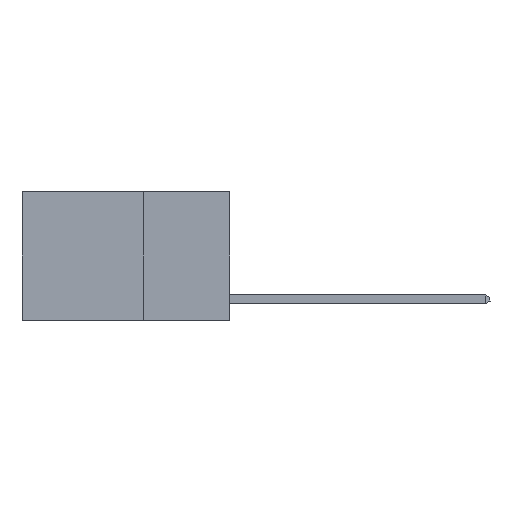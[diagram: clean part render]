
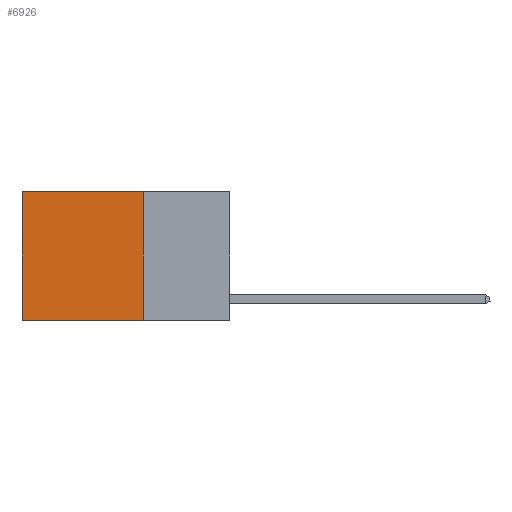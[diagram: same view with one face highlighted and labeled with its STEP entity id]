
A CAD part, left-side view. The second image highlights one B-rep face of the part: STEP entity #6926.
In plain terms, the highlighted planar face has unit normal (-1, 0, 0).
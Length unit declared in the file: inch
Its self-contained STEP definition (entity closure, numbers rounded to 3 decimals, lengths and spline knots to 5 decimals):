
#720 = LINE ( 'NONE', #11697, #869 ) ;
#869 = VECTOR ( 'NONE', #1500, 39.37008 ) ;
#1333 = LINE ( 'NONE', #8462, #12494 ) ;
#1369 = PLANE ( 'NONE',  #10011 ) ;
#1450 = DIRECTION ( 'NONE',  ( 0., 0., -1. ) ) ;
#1488 = LINE ( 'NONE', #3428, #2907 ) ;
#1500 = DIRECTION ( 'NONE',  ( 0., 0., -1. ) ) ;
#1533 = CARTESIAN_POINT ( 'NONE',  ( 0.2625, 0.25, 0. ) ) ;
#1823 = EDGE_CURVE ( 'NONE', #12910, #5842, #720, .T. ) ;
#2907 = VECTOR ( 'NONE', #11552, 39.37008 ) ;
#3292 = EDGE_CURVE ( 'NONE', #6196, #12910, #1488, .T. ) ;
#3428 = CARTESIAN_POINT ( 'NONE',  ( 0.2625, 0.25, 0. ) ) ;
#3432 = CARTESIAN_POINT ( 'NONE',  ( 0.2625, 0.25, 0. ) ) ;
#3776 = CARTESIAN_POINT ( 'NONE',  ( 0.2625, 0.6, 0. ) ) ;
#4314 = VECTOR ( 'NONE', #1450, 39.37008 ) ;
#4449 = CARTESIAN_POINT ( 'NONE',  ( 0.2625, 0.25, 0. ) ) ;
#5058 = CARTESIAN_POINT ( 'NONE',  ( 0.2625, 0.25, -0.37 ) ) ;
#5737 = ORIENTED_EDGE ( 'NONE', *, *, #1823, .T. ) ;
#5842 = VERTEX_POINT ( 'NONE', #6462 ) ;
#6196 = VERTEX_POINT ( 'NONE', #1533 ) ;
#6462 = CARTESIAN_POINT ( 'NONE',  ( 0.2625, 0.6, -0.37 ) ) ;
#6736 = EDGE_LOOP ( 'NONE', ( #5737, #9931, #10718, #8249 ) ) ;
#6926 = ADVANCED_FACE ( 'NONE', ( #11349 ), #1369, .F. ) ;
#8249 = ORIENTED_EDGE ( 'NONE', *, *, #3292, .T. ) ;
#8462 = CARTESIAN_POINT ( 'NONE',  ( 0.2625, 0.25, -0.37 ) ) ;
#9570 = EDGE_CURVE ( 'NONE', #6196, #11566, #12366, .T. ) ;
#9606 = EDGE_CURVE ( 'NONE', #11566, #5842, #1333, .T. ) ;
#9931 = ORIENTED_EDGE ( 'NONE', *, *, #9606, .F. ) ;
#10011 = AXIS2_PLACEMENT_3D ( 'NONE', #3432, #12468, #12406 ) ;
#10718 = ORIENTED_EDGE ( 'NONE', *, *, #9570, .F. ) ;
#11185 = DIRECTION ( 'NONE',  ( 0., 1., 0. ) ) ;
#11349 = FACE_OUTER_BOUND ( 'NONE', #6736, .T. ) ;
#11552 = DIRECTION ( 'NONE',  ( 0., 1., 0. ) ) ;
#11566 = VERTEX_POINT ( 'NONE', #5058 ) ;
#11697 = CARTESIAN_POINT ( 'NONE',  ( 0.2625, 0.6, 0. ) ) ;
#12366 = LINE ( 'NONE', #4449, #4314 ) ;
#12406 = DIRECTION ( 'NONE',  ( 0., 0., -1. ) ) ;
#12468 = DIRECTION ( 'NONE',  ( 1., 0., 0. ) ) ;
#12494 = VECTOR ( 'NONE', #11185, 39.37008 ) ;
#12910 = VERTEX_POINT ( 'NONE', #3776 ) ;
